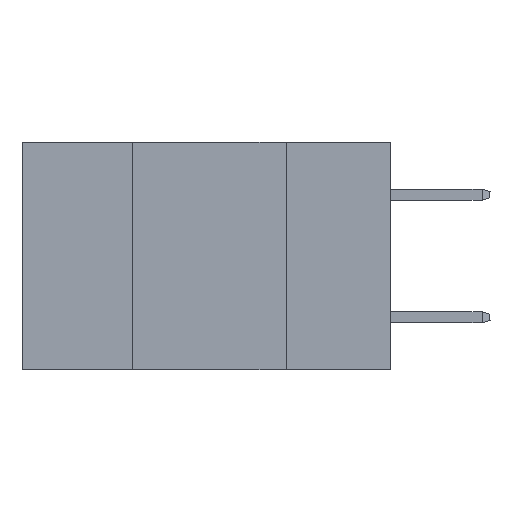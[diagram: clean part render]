
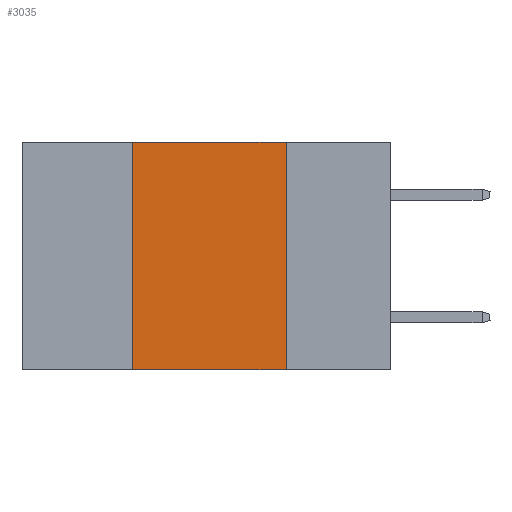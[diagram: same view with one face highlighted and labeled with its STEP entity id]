
A CAD part, left-side view. The second image highlights one B-rep face of the part: STEP entity #3035.
In plain terms, the highlighted planar face has unit normal (-1, 0, 0).
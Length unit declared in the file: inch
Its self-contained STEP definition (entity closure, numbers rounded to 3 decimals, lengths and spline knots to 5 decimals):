
#19 = VECTOR ( 'NONE', #7210, 39.37008 ) ;
#392 = CARTESIAN_POINT ( 'NONE',  ( 0., 0.6, 0. ) ) ;
#412 = CARTESIAN_POINT ( 'NONE',  ( 0., 0.17, -0.37 ) ) ;
#847 = DIRECTION ( 'NONE',  ( 1., 0., 0. ) ) ;
#860 = DIRECTION ( 'NONE',  ( 0., 0., -1. ) ) ;
#872 = PLANE ( 'NONE',  #2932 ) ;
#1886 = CARTESIAN_POINT ( 'NONE',  ( 0., 0.6, -0.37 ) ) ;
#2183 = EDGE_LOOP ( 'NONE', ( #6381, #6579, #6813, #7041 ) ) ;
#2582 = EDGE_CURVE ( 'NONE', #4092, #6839, #6865, .T. ) ;
#2626 = EDGE_CURVE ( 'NONE', #6839, #7507, #10050, .T. ) ;
#2724 = EDGE_CURVE ( 'NONE', #7507, #5803, #3486, .T. ) ;
#2932 = AXIS2_PLACEMENT_3D ( 'NONE', #392, #847, #860 ) ;
#3035 = ADVANCED_FACE ( 'NONE', ( #6611 ), #872, .F. ) ;
#3486 = LINE ( 'NONE', #4364, #5393 ) ;
#4092 = VERTEX_POINT ( 'NONE', #5416 ) ;
#4364 = CARTESIAN_POINT ( 'NONE',  ( 0., 0.17, 0. ) ) ;
#4423 = CARTESIAN_POINT ( 'NONE',  ( 0., 0.6, 0. ) ) ;
#4438 = DIRECTION ( 'NONE',  ( 0., -1., 0. ) ) ;
#4506 = DIRECTION ( 'NONE',  ( 0., 0., -1. ) ) ;
#4540 = DIRECTION ( 'NONE',  ( 0., -1., 0. ) ) ;
#5393 = VECTOR ( 'NONE', #4506, 39.37008 ) ;
#5416 = CARTESIAN_POINT ( 'NONE',  ( 0., 0.42, -0.37 ) ) ;
#5803 = VERTEX_POINT ( 'NONE', #412 ) ;
#5814 = CARTESIAN_POINT ( 'NONE',  ( 0., 0.17, 0. ) ) ;
#6097 = LINE ( 'NONE', #1886, #9566 ) ;
#6381 = ORIENTED_EDGE ( 'NONE', *, *, #2724, .F. ) ;
#6384 = VECTOR ( 'NONE', #4438, 39.37008 ) ;
#6579 = ORIENTED_EDGE ( 'NONE', *, *, #2626, .F. ) ;
#6611 = FACE_OUTER_BOUND ( 'NONE', #2183, .T. ) ;
#6721 = CARTESIAN_POINT ( 'NONE',  ( 0., 0.42, 0. ) ) ;
#6813 = ORIENTED_EDGE ( 'NONE', *, *, #2582, .F. ) ;
#6839 = VERTEX_POINT ( 'NONE', #6721 ) ;
#6865 = LINE ( 'NONE', #6981, #19 ) ;
#6981 = CARTESIAN_POINT ( 'NONE',  ( 0., 0.42, 0. ) ) ;
#7041 = ORIENTED_EDGE ( 'NONE', *, *, #9363, .T. ) ;
#7210 = DIRECTION ( 'NONE',  ( 0., 0., 1. ) ) ;
#7507 = VERTEX_POINT ( 'NONE', #5814 ) ;
#9363 = EDGE_CURVE ( 'NONE', #4092, #5803, #6097, .T. ) ;
#9566 = VECTOR ( 'NONE', #4540, 39.37008 ) ;
#10050 = LINE ( 'NONE', #4423, #6384 ) ;
